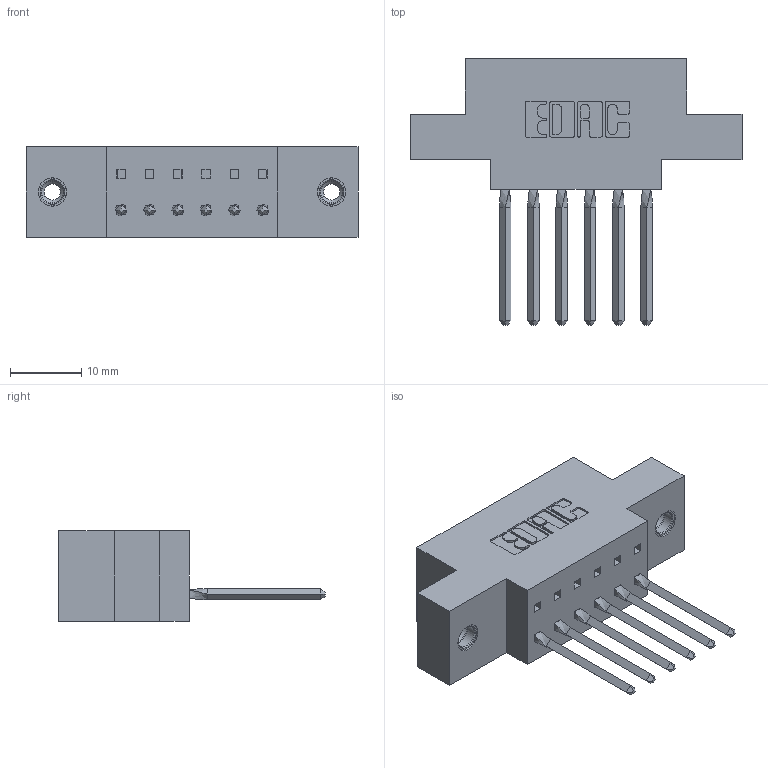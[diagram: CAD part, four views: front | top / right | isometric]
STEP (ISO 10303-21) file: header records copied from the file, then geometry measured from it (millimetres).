
FILE_DESCRIPTION (( 'STEP AP203' ), '1' );
FILE_NAME ('317-006-541-678.STEP', '2020-02-27T12:48:26', ( '' ), ( '' ), 'SwSTEP 2.0', 'SolidWorks 2016', '' );
FILE_SCHEMA (( 'CONFIG_CONTROL_DESIGN' ));
Length unit declared in the file: inch
Products named in the file (4): 345-250-001_345-250-003-102; 317-290-002_541; 317 Part_.156 Dia - TI; 317-006-541-678
Assembly tree (9 placements, depth 2):
  317-006-541-678
    317 Part_.156 Dia - TI
    317-290-002_541  x6
    345-250-001_345-250-003-102  x2
Bounding box: 46.48 x 37.34 x 12.7 mm (x, y, z)
Volume: 6424.4 mm3; surface area: 7899.4 mm2
Topology: 9 solids, 9 shells, 1074 faces, 3015 edges, 1958 vertices
Faces by surface type: plane 834, cylinder 200, bspline 24, cone 12, torus 4
Entity records: 16237 total; most frequent: CARTESIAN_POINT 3478, ORIENTED_EDGE 2730, DIRECTION 2259, EDGE_CURVE 1365, VECTOR 981, LINE 981, VERTEX_POINT 898, AXIS2_PLACEMENT_3D 639
